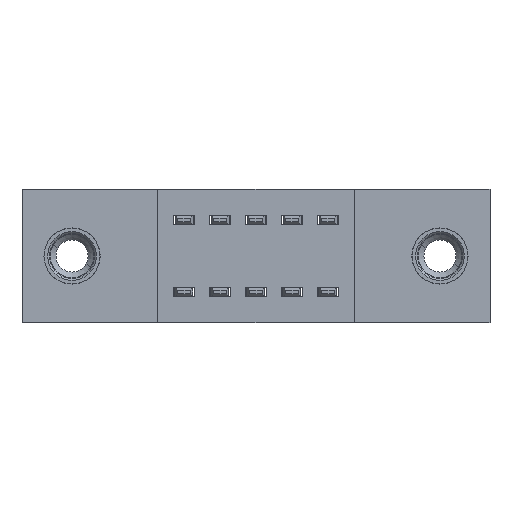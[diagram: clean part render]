
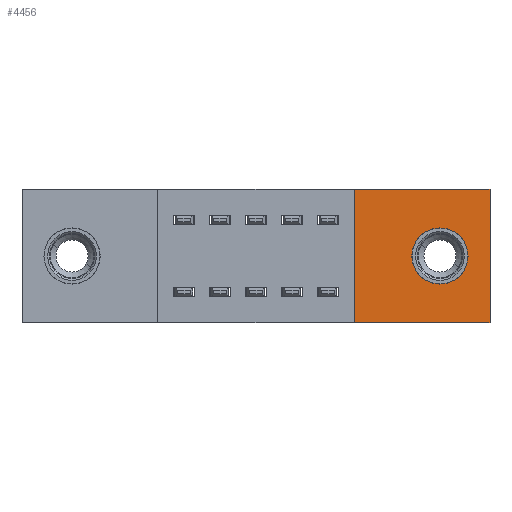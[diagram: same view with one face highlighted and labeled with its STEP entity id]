
A CAD part, front view. The second image highlights one B-rep face of the part: STEP entity #4456.
In plain terms, the highlighted planar face has unit normal (0, -1, 0).
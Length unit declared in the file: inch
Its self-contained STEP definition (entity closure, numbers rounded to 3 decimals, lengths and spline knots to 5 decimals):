
#328 = CARTESIAN_POINT ( 'NONE',  ( 1.161, 0., -0.185 ) ) ;
#456 = ORIENTED_EDGE ( 'NONE', *, *, #2402, .F. ) ;
#662 = LINE ( 'NONE', #5717, #883 ) ;
#722 = CARTESIAN_POINT ( 'NONE',  ( 1.3, 0., -0.37 ) ) ;
#883 = VECTOR ( 'NONE', #2305, 39.37008 ) ;
#960 = EDGE_LOOP ( 'NONE', ( #1381, #2767 ) ) ;
#1008 = DIRECTION ( 'NONE',  ( 0., 0., -1. ) ) ;
#1176 = ORIENTED_EDGE ( 'NONE', *, *, #7880, .F. ) ;
#1226 = VECTOR ( 'NONE', #7956, 39.37008 ) ;
#1381 = ORIENTED_EDGE ( 'NONE', *, *, #6231, .T. ) ;
#1518 = VERTEX_POINT ( 'NONE', #8313 ) ;
#1587 = DIRECTION ( 'NONE',  ( 0., 1., 0. ) ) ;
#1600 = VERTEX_POINT ( 'NONE', #722 ) ;
#1833 = VERTEX_POINT ( 'NONE', #2871 ) ;
#2210 = LINE ( 'NONE', #4151, #7488 ) ;
#2305 = DIRECTION ( 'NONE',  ( 0., 0., 1. ) ) ;
#2402 = EDGE_CURVE ( 'NONE', #5842, #1833, #662, .T. ) ;
#2767 = ORIENTED_EDGE ( 'NONE', *, *, #8605, .T. ) ;
#2871 = CARTESIAN_POINT ( 'NONE',  ( 0.923, 0., 0. ) ) ;
#2872 = FACE_OUTER_BOUND ( 'NONE', #4720, .T. ) ;
#3039 = CARTESIAN_POINT ( 'NONE',  ( 0., 0., -0.37 ) ) ;
#3251 = LINE ( 'NONE', #8612, #1226 ) ;
#3254 = AXIS2_PLACEMENT_3D ( 'NONE', #5693, #1587, #6376 ) ;
#3485 = DIRECTION ( 'NONE',  ( 0., 0., -1. ) ) ;
#3721 = DIRECTION ( 'NONE',  ( 0., -1., 0. ) ) ;
#3841 = CARTESIAN_POINT ( 'NONE',  ( 1.161, 0., -0.263 ) ) ;
#4151 = CARTESIAN_POINT ( 'NONE',  ( 1.3, 0., 0. ) ) ;
#4228 = DIRECTION ( 'NONE',  ( 1., 0., 0. ) ) ;
#4456 = ADVANCED_FACE ( 'NONE', ( #6307, #2872 ), #7171, .T. ) ;
#4573 = VERTEX_POINT ( 'NONE', #3841 ) ;
#4655 = CIRCLE ( 'NONE', #3254, 0.078 ) ;
#4720 = EDGE_LOOP ( 'NONE', ( #456, #6533, #1176, #5939 ) ) ;
#5103 = DIRECTION ( 'NONE',  ( 0., 1., 0. ) ) ;
#5673 = AXIS2_PLACEMENT_3D ( 'NONE', #3039, #3721, #8554 ) ;
#5693 = CARTESIAN_POINT ( 'NONE',  ( 1.161, 0., -0.185 ) ) ;
#5717 = CARTESIAN_POINT ( 'NONE',  ( 0.923, 0., -0.37 ) ) ;
#5842 = VERTEX_POINT ( 'NONE', #8063 ) ;
#5939 = ORIENTED_EDGE ( 'NONE', *, *, #7223, .F. ) ;
#6231 = EDGE_CURVE ( 'NONE', #1518, #4573, #4655, .T. ) ;
#6271 = CARTESIAN_POINT ( 'NONE',  ( 0., 0., 0. ) ) ;
#6307 = FACE_BOUND ( 'NONE', #960, .T. ) ;
#6376 = DIRECTION ( 'NONE',  ( 0., 0., -1. ) ) ;
#6533 = ORIENTED_EDGE ( 'NONE', *, *, #8678, .F. ) ;
#7036 = VECTOR ( 'NONE', #4228, 39.37008 ) ;
#7171 = PLANE ( 'NONE',  #5673 ) ;
#7223 = EDGE_CURVE ( 'NONE', #1833, #7736, #8874, .T. ) ;
#7367 = CIRCLE ( 'NONE', #8866, 0.078 ) ;
#7488 = VECTOR ( 'NONE', #3485, 39.37008 ) ;
#7736 = VERTEX_POINT ( 'NONE', #8148 ) ;
#7880 = EDGE_CURVE ( 'NONE', #7736, #1600, #2210, .T. ) ;
#7956 = DIRECTION ( 'NONE',  ( -1., 0., 0. ) ) ;
#8063 = CARTESIAN_POINT ( 'NONE',  ( 0.923, 0., -0.37 ) ) ;
#8148 = CARTESIAN_POINT ( 'NONE',  ( 1.3, 0., 0. ) ) ;
#8313 = CARTESIAN_POINT ( 'NONE',  ( 1.161, 0., -0.107 ) ) ;
#8554 = DIRECTION ( 'NONE',  ( 0., 0., -1. ) ) ;
#8605 = EDGE_CURVE ( 'NONE', #4573, #1518, #7367, .T. ) ;
#8612 = CARTESIAN_POINT ( 'NONE',  ( 0., 0., -0.37 ) ) ;
#8678 = EDGE_CURVE ( 'NONE', #1600, #5842, #3251, .T. ) ;
#8866 = AXIS2_PLACEMENT_3D ( 'NONE', #328, #5103, #1008 ) ;
#8874 = LINE ( 'NONE', #6271, #7036 ) ;
